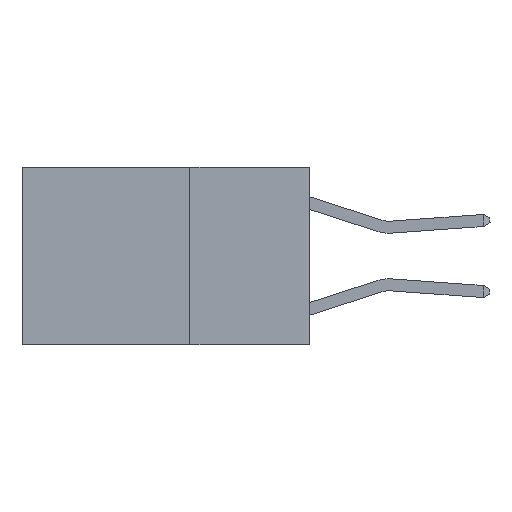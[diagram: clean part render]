
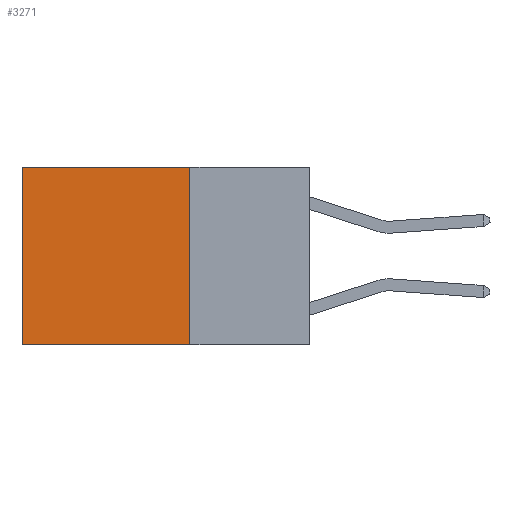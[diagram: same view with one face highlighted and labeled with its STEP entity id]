
A CAD part, left-side view. The second image highlights one B-rep face of the part: STEP entity #3271.
In plain terms, the highlighted planar face has unit normal (-1, 0, 0).
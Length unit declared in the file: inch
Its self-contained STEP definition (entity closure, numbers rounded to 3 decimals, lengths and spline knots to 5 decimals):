
#103 = CARTESIAN_POINT ( 'NONE',  ( 0.2625, 0.25, 0. ) ) ;
#752 = CARTESIAN_POINT ( 'NONE',  ( 0.2625, 0.25, -0.37 ) ) ;
#848 = DIRECTION ( 'NONE',  ( 0., 1., 0. ) ) ;
#969 = LINE ( 'NONE', #7905, #7081 ) ;
#1529 = LINE ( 'NONE', #103, #8018 ) ;
#1810 = DIRECTION ( 'NONE',  ( 0., 1., 0. ) ) ;
#2131 = LINE ( 'NONE', #11828, #11459 ) ;
#2917 = EDGE_CURVE ( 'NONE', #3540, #13461, #969, .T. ) ;
#3067 = EDGE_CURVE ( 'NONE', #8961, #15193, #2131, .T. ) ;
#3271 = ADVANCED_FACE ( 'NONE', ( #5966 ), #7312, .F. ) ;
#3540 = VERTEX_POINT ( 'NONE', #6772 ) ;
#3781 = DIRECTION ( 'NONE',  ( 0., 0., -1. ) ) ;
#5329 = ORIENTED_EDGE ( 'NONE', *, *, #3067, .F. ) ;
#5776 = CARTESIAN_POINT ( 'NONE',  ( 0.2625, 0.6, -0.37 ) ) ;
#5966 = FACE_OUTER_BOUND ( 'NONE', #9524, .T. ) ;
#6661 = LINE ( 'NONE', #7482, #10667 ) ;
#6772 = CARTESIAN_POINT ( 'NONE',  ( 0.2625, 0.25, 0. ) ) ;
#7081 = VECTOR ( 'NONE', #1810, 39.37008 ) ;
#7312 = PLANE ( 'NONE',  #13300 ) ;
#7482 = CARTESIAN_POINT ( 'NONE',  ( 0.2625, 0.6, 0. ) ) ;
#7905 = CARTESIAN_POINT ( 'NONE',  ( 0.2625, 0.25, 0. ) ) ;
#7995 = ORIENTED_EDGE ( 'NONE', *, *, #2917, .T. ) ;
#8018 = VECTOR ( 'NONE', #8651, 39.37008 ) ;
#8524 = DIRECTION ( 'NONE',  ( 0., 0., -1. ) ) ;
#8651 = DIRECTION ( 'NONE',  ( 0., 0., -1. ) ) ;
#8961 = VERTEX_POINT ( 'NONE', #752 ) ;
#9524 = EDGE_LOOP ( 'NONE', ( #15326, #5329, #14017, #7995 ) ) ;
#9696 = CARTESIAN_POINT ( 'NONE',  ( 0.2625, 0.25, 0. ) ) ;
#10667 = VECTOR ( 'NONE', #3781, 39.37008 ) ;
#10689 = CARTESIAN_POINT ( 'NONE',  ( 0.2625, 0.6, 0. ) ) ;
#11459 = VECTOR ( 'NONE', #848, 39.37008 ) ;
#11618 = DIRECTION ( 'NONE',  ( 1., 0., 0. ) ) ;
#11753 = EDGE_CURVE ( 'NONE', #3540, #8961, #1529, .T. ) ;
#11828 = CARTESIAN_POINT ( 'NONE',  ( 0.2625, 0.25, -0.37 ) ) ;
#12492 = EDGE_CURVE ( 'NONE', #13461, #15193, #6661, .T. ) ;
#13300 = AXIS2_PLACEMENT_3D ( 'NONE', #9696, #11618, #8524 ) ;
#13461 = VERTEX_POINT ( 'NONE', #10689 ) ;
#14017 = ORIENTED_EDGE ( 'NONE', *, *, #11753, .F. ) ;
#15193 = VERTEX_POINT ( 'NONE', #5776 ) ;
#15326 = ORIENTED_EDGE ( 'NONE', *, *, #12492, .T. ) ;
